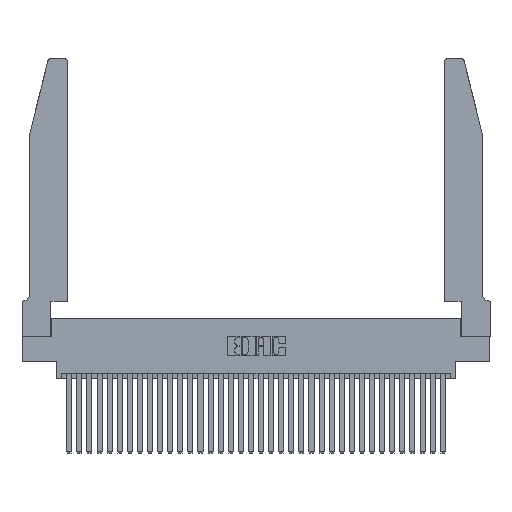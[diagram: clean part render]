
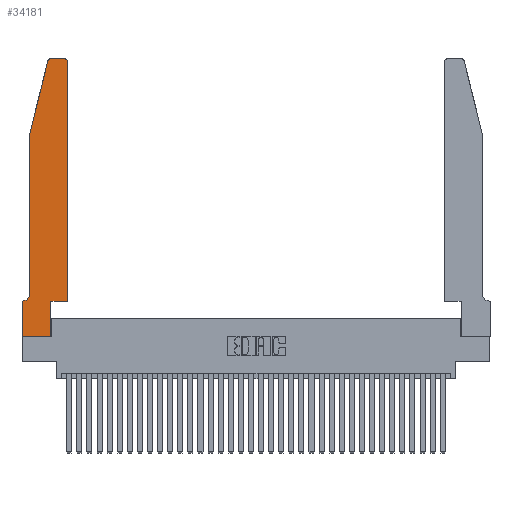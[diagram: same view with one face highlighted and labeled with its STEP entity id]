
A CAD part, top view. The second image highlights one B-rep face of the part: STEP entity #34181.
In plain terms, the highlighted planar face has unit normal (0, 0, 1).
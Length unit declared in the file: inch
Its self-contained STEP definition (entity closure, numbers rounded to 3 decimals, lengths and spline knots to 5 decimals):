
#271 = CARTESIAN_POINT ( 'NONE',  ( 0.2605, 2.75, 0.37 ) ) ;
#470 = VERTEX_POINT ( 'NONE', #32254 ) ;
#502 = DIRECTION ( 'NONE',  ( 0., 0., 1. ) ) ;
#591 = CARTESIAN_POINT ( 'NONE',  ( 0.4205, 2.75, 0.37 ) ) ;
#914 = EDGE_LOOP ( 'NONE', ( #29740, #2060, #19983, #28671, #28845, #20538, #13617, #11218, #23565, #34693, #33733, #11617 ) ) ;
#1012 = CARTESIAN_POINT ( 'NONE',  ( 0.0055, 0.35, 0.37 ) ) ;
#2060 = ORIENTED_EDGE ( 'NONE', *, *, #27017, .T. ) ;
#2082 = CARTESIAN_POINT ( 'NONE',  ( 0.0755, 2., 0.37 ) ) ;
#2109 = CARTESIAN_POINT ( 'NONE',  ( 0.284, 2.75, 0.37 ) ) ;
#2598 = DIRECTION ( 'NONE',  ( 1., 0., 0. ) ) ;
#2682 = VERTEX_POINT ( 'NONE', #2109 ) ;
#2981 = CARTESIAN_POINT ( 'NONE',  ( 0.0055, 0.42, 0.37 ) ) ;
#3463 = LINE ( 'NONE', #20213, #31409 ) ;
#3531 = VECTOR ( 'NONE', #2598, 39.37008 ) ;
#3833 = VERTEX_POINT ( 'NONE', #25806 ) ;
#4136 = AXIS2_PLACEMENT_3D ( 'NONE', #27591, #502, #19502 ) ;
#4183 = DIRECTION ( 'NONE',  ( 0., 0., 1. ) ) ;
#4328 = CARTESIAN_POINT ( 'NONE',  ( 0.2865, 0., 0.37 ) ) ;
#4482 = AXIS2_PLACEMENT_3D ( 'NONE', #20463, #4183, #23196 ) ;
#4711 = VECTOR ( 'NONE', #7342, 39.37008 ) ;
#4872 = CIRCLE ( 'NONE', #4482, 0.03 ) ;
#4935 = LINE ( 'NONE', #16053, #30365 ) ;
#5365 = CARTESIAN_POINT ( 'NONE',  ( 0.0755, 0.42, 0.37 ) ) ;
#5685 = DIRECTION ( 'NONE',  ( -1., 0., 0. ) ) ;
#5883 = VERTEX_POINT ( 'NONE', #4328 ) ;
#6693 = VERTEX_POINT ( 'NONE', #23904 ) ;
#6825 = AXIS2_PLACEMENT_3D ( 'NONE', #2981, #21985, #5685 ) ;
#7342 = DIRECTION ( 'NONE',  ( 1., 0., 0. ) ) ;
#8000 = DIRECTION ( 'NONE',  ( 0., 1., 0. ) ) ;
#8095 = CARTESIAN_POINT ( 'NONE',  ( 0., 0.35, 0.37 ) ) ;
#8204 = CIRCLE ( 'NONE', #6825, 0.07 ) ;
#10120 = LINE ( 'NONE', #271, #22053 ) ;
#10204 = VERTEX_POINT ( 'NONE', #33771 ) ;
#10401 = VECTOR ( 'NONE', #18154, 39.37008 ) ;
#11218 = ORIENTED_EDGE ( 'NONE', *, *, #26880, .T. ) ;
#11367 = CARTESIAN_POINT ( 'NONE',  ( 0.284, 2.72, 0.37 ) ) ;
#11617 = ORIENTED_EDGE ( 'NONE', *, *, #15944, .T. ) ;
#11961 = AXIS2_PLACEMENT_3D ( 'NONE', #11367, #30308, #14084 ) ;
#12705 = VERTEX_POINT ( 'NONE', #1012 ) ;
#12765 = LINE ( 'NONE', #20919, #4711 ) ;
#13034 = VECTOR ( 'NONE', #31511, 39.37008 ) ;
#13050 = VERTEX_POINT ( 'NONE', #5365 ) ;
#13617 = ORIENTED_EDGE ( 'NONE', *, *, #21306, .T. ) ;
#13814 = DIRECTION ( 'NONE',  ( -1., 0., 0. ) ) ;
#14084 = DIRECTION ( 'NONE',  ( 1., 0., 0. ) ) ;
#15127 = EDGE_CURVE ( 'NONE', #470, #3833, #4935, .T. ) ;
#15944 = EDGE_CURVE ( 'NONE', #3833, #28305, #4872, .T. ) ;
#16053 = CARTESIAN_POINT ( 'NONE',  ( 0.4505, 0.35, 0.37 ) ) ;
#17177 = VECTOR ( 'NONE', #25614, 39.37008 ) ;
#18154 = DIRECTION ( 'NONE',  ( 0., 1., 0. ) ) ;
#19502 = DIRECTION ( 'NONE',  ( 1., 0., 0. ) ) ;
#19983 = ORIENTED_EDGE ( 'NONE', *, *, #31982, .T. ) ;
#20213 = CARTESIAN_POINT ( 'NONE',  ( 0.0755, 0.35, 0.37 ) ) ;
#20284 = LINE ( 'NONE', #23418, #13034 ) ;
#20368 = EDGE_CURVE ( 'NONE', #28305, #2682, #10120, .T. ) ;
#20463 = CARTESIAN_POINT ( 'NONE',  ( 0.4205, 2.72, 0.37 ) ) ;
#20538 = ORIENTED_EDGE ( 'NONE', *, *, #27819, .T. ) ;
#20891 = VECTOR ( 'NONE', #31918, 39.37008 ) ;
#20919 = CARTESIAN_POINT ( 'NONE',  ( 0.4505, 0.35, 0.37 ) ) ;
#21052 = CARTESIAN_POINT ( 'NONE',  ( 0.25487, 2.72718, 0.37 ) ) ;
#21306 = EDGE_CURVE ( 'NONE', #27595, #10204, #20284, .T. ) ;
#21985 = DIRECTION ( 'NONE',  ( 0., 0., -1. ) ) ;
#22053 = VECTOR ( 'NONE', #13814, 39.37008 ) ;
#22690 = VERTEX_POINT ( 'NONE', #21052 ) ;
#22883 = CARTESIAN_POINT ( 'NONE',  ( 0.0755, 2., 0.37 ) ) ;
#23196 = DIRECTION ( 'NONE',  ( 1., 0., 0. ) ) ;
#23418 = CARTESIAN_POINT ( 'NONE',  ( 0., 0., 0.37 ) ) ;
#23565 = ORIENTED_EDGE ( 'NONE', *, *, #32193, .T. ) ;
#23904 = CARTESIAN_POINT ( 'NONE',  ( 0.2865, 0.35, 0.37 ) ) ;
#25339 = FACE_OUTER_BOUND ( 'NONE', #914, .T. ) ;
#25614 = DIRECTION ( 'NONE',  ( -0.239, -0.971, 0. ) ) ;
#25725 = LINE ( 'NONE', #31659, #10401 ) ;
#25806 = CARTESIAN_POINT ( 'NONE',  ( 0.4505, 2.72, 0.37 ) ) ;
#26880 = EDGE_CURVE ( 'NONE', #10204, #5883, #31475, .T. ) ;
#26967 = VERTEX_POINT ( 'NONE', #29960 ) ;
#27017 = EDGE_CURVE ( 'NONE', #2682, #22690, #27297, .T. ) ;
#27297 = CIRCLE ( 'NONE', #11961, 0.03 ) ;
#27453 = EDGE_CURVE ( 'NONE', #26967, #13050, #28110, .T. ) ;
#27591 = CARTESIAN_POINT ( 'NONE',  ( 0., 0.35, 0.37 ) ) ;
#27595 = VERTEX_POINT ( 'NONE', #8095 ) ;
#27819 = EDGE_CURVE ( 'NONE', #12705, #27595, #3463, .T. ) ;
#27984 = EDGE_CURVE ( 'NONE', #6693, #470, #12765, .T. ) ;
#28110 = LINE ( 'NONE', #2082, #20891 ) ;
#28305 = VERTEX_POINT ( 'NONE', #591 ) ;
#28388 = DIRECTION ( 'NONE',  ( -1., 0., 0. ) ) ;
#28671 = ORIENTED_EDGE ( 'NONE', *, *, #27453, .T. ) ;
#28845 = ORIENTED_EDGE ( 'NONE', *, *, #32934, .T. ) ;
#29608 = CARTESIAN_POINT ( 'NONE',  ( 0., 0., 0.37 ) ) ;
#29740 = ORIENTED_EDGE ( 'NONE', *, *, #20368, .T. ) ;
#29960 = CARTESIAN_POINT ( 'NONE',  ( 0.0755, 2., 0.37 ) ) ;
#30308 = DIRECTION ( 'NONE',  ( 0., 0., 1. ) ) ;
#30365 = VECTOR ( 'NONE', #8000, 39.37008 ) ;
#31409 = VECTOR ( 'NONE', #28388, 39.37008 ) ;
#31475 = LINE ( 'NONE', #29608, #3531 ) ;
#31511 = DIRECTION ( 'NONE',  ( 0., -1., 0. ) ) ;
#31585 = LINE ( 'NONE', #22883, #17177 ) ;
#31659 = CARTESIAN_POINT ( 'NONE',  ( 0.2865, 0.35, 0.37 ) ) ;
#31918 = DIRECTION ( 'NONE',  ( 0., -1., 0. ) ) ;
#31982 = EDGE_CURVE ( 'NONE', #22690, #26967, #31585, .T. ) ;
#32193 = EDGE_CURVE ( 'NONE', #5883, #6693, #25725, .T. ) ;
#32254 = CARTESIAN_POINT ( 'NONE',  ( 0.4505, 0.35, 0.37 ) ) ;
#32934 = EDGE_CURVE ( 'NONE', #13050, #12705, #8204, .T. ) ;
#32962 = PLANE ( 'NONE',  #4136 ) ;
#33733 = ORIENTED_EDGE ( 'NONE', *, *, #15127, .T. ) ;
#33771 = CARTESIAN_POINT ( 'NONE',  ( 0., 0., 0.37 ) ) ;
#34181 = ADVANCED_FACE ( 'NONE', ( #25339 ), #32962, .T. ) ;
#34693 = ORIENTED_EDGE ( 'NONE', *, *, #27984, .T. ) ;
